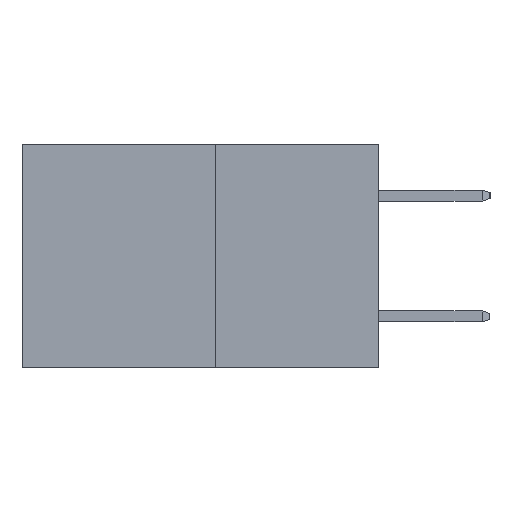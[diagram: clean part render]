
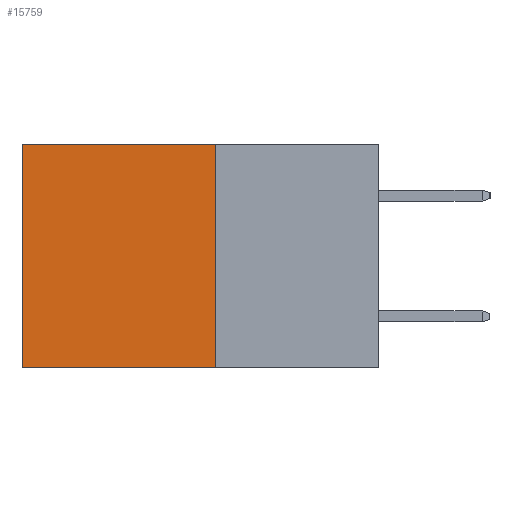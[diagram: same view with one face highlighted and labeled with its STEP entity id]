
A CAD part, left-side view. The second image highlights one B-rep face of the part: STEP entity #15759.
In plain terms, the highlighted planar face has unit normal (-1, 0, 0).
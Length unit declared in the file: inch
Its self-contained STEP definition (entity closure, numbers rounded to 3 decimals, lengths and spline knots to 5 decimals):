
#48 = DIRECTION ( 'NONE',  ( 0., 1., 0. ) ) ;
#130 = ORIENTED_EDGE ( 'NONE', *, *, #8910, .T. ) ;
#1006 = VERTEX_POINT ( 'NONE', #5337 ) ;
#1816 = EDGE_CURVE ( 'NONE', #9930, #11991, #17124, .T. ) ;
#2251 = VECTOR ( 'NONE', #13011, 39.37008 ) ;
#3747 = DIRECTION ( 'NONE',  ( 0., 1., 0. ) ) ;
#5337 = CARTESIAN_POINT ( 'NONE',  ( 0.277, 0.59, 0. ) ) ;
#5809 = CARTESIAN_POINT ( 'NONE',  ( 0.277, 0.59, -0.37 ) ) ;
#6063 = DIRECTION ( 'NONE',  ( 0., 0., -1. ) ) ;
#7815 = CARTESIAN_POINT ( 'NONE',  ( 0.277, 0.27, -0.37 ) ) ;
#8398 = ORIENTED_EDGE ( 'NONE', *, *, #19069, .T. ) ;
#8655 = CARTESIAN_POINT ( 'NONE',  ( 0.277, 0.27, -0.37 ) ) ;
#8910 = EDGE_CURVE ( 'NONE', #12019, #1006, #15896, .T. ) ;
#8917 = ORIENTED_EDGE ( 'NONE', *, *, #15495, .F. ) ;
#9930 = VERTEX_POINT ( 'NONE', #7815 ) ;
#10235 = CARTESIAN_POINT ( 'NONE',  ( 0.277, 0.27, -0.37 ) ) ;
#10332 = DIRECTION ( 'NONE',  ( 0., 0., -1. ) ) ;
#10456 = VECTOR ( 'NONE', #6063, 39.37008 ) ;
#11991 = VERTEX_POINT ( 'NONE', #5809 ) ;
#12019 = VERTEX_POINT ( 'NONE', #20874 ) ;
#13011 = DIRECTION ( 'NONE',  ( 0., 0., -1. ) ) ;
#13900 = CARTESIAN_POINT ( 'NONE',  ( 0.277, 0.27, 0. ) ) ;
#14501 = FACE_OUTER_BOUND ( 'NONE', #16853, .T. ) ;
#15294 = PLANE ( 'NONE',  #18599 ) ;
#15495 = EDGE_CURVE ( 'NONE', #12019, #9930, #16352, .T. ) ;
#15759 = ADVANCED_FACE ( 'NONE', ( #14501 ), #15294, .F. ) ;
#15896 = LINE ( 'NONE', #13900, #20292 ) ;
#15965 = LINE ( 'NONE', #16142, #10456 ) ;
#16142 = CARTESIAN_POINT ( 'NONE',  ( 0.277, 0.59, -0.37 ) ) ;
#16352 = LINE ( 'NONE', #19659, #2251 ) ;
#16853 = EDGE_LOOP ( 'NONE', ( #8398, #17262, #8917, #130 ) ) ;
#16893 = VECTOR ( 'NONE', #48, 39.37008 ) ;
#17124 = LINE ( 'NONE', #10235, #16893 ) ;
#17262 = ORIENTED_EDGE ( 'NONE', *, *, #1816, .F. ) ;
#18599 = AXIS2_PLACEMENT_3D ( 'NONE', #8655, #20306, #10332 ) ;
#19069 = EDGE_CURVE ( 'NONE', #1006, #11991, #15965, .T. ) ;
#19659 = CARTESIAN_POINT ( 'NONE',  ( 0.277, 0.27, -0.37 ) ) ;
#20292 = VECTOR ( 'NONE', #3747, 39.37008 ) ;
#20306 = DIRECTION ( 'NONE',  ( 1., 0., 0. ) ) ;
#20874 = CARTESIAN_POINT ( 'NONE',  ( 0.277, 0.27, 0. ) ) ;
